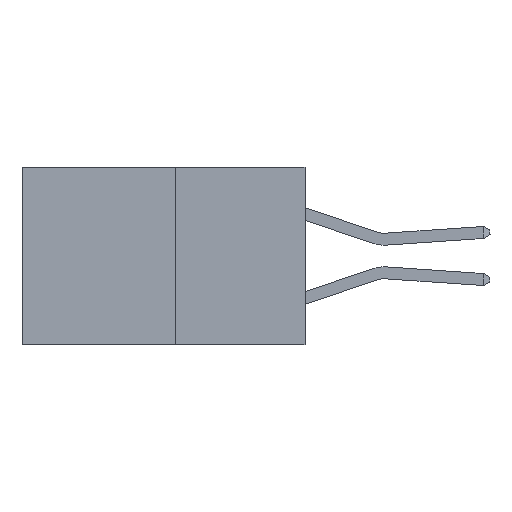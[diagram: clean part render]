
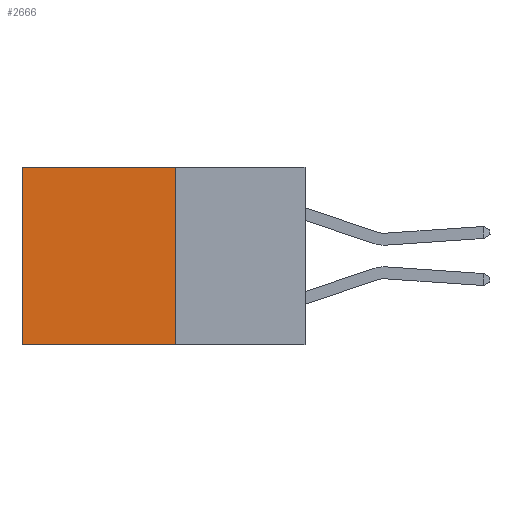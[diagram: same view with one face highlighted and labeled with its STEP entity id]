
A CAD part, left-side view. The second image highlights one B-rep face of the part: STEP entity #2666.
In plain terms, the highlighted planar face has unit normal (-1, 0, 0).
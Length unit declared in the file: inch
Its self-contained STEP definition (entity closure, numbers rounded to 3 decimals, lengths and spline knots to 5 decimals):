
#47 = CARTESIAN_POINT ( 'NONE',  ( 0.277, 0.27, -0.37 ) ) ;
#79 = CARTESIAN_POINT ( 'NONE',  ( 0.277, 0.27, -0.37 ) ) ;
#841 = LINE ( 'NONE', #14643, #8844 ) ;
#1040 = DIRECTION ( 'NONE',  ( 1., 0., 0. ) ) ;
#1284 = VERTEX_POINT ( 'NONE', #3802 ) ;
#1543 = VECTOR ( 'NONE', #5683, 39.37008 ) ;
#1975 = CARTESIAN_POINT ( 'NONE',  ( 0.277, 0.59, -0.37 ) ) ;
#2591 = ORIENTED_EDGE ( 'NONE', *, *, #8512, .T. ) ;
#2666 = ADVANCED_FACE ( 'NONE', ( #12675 ), #11684, .F. ) ;
#3070 = ORIENTED_EDGE ( 'NONE', *, *, #3448, .T. ) ;
#3448 = EDGE_CURVE ( 'NONE', #5344, #10267, #841, .T. ) ;
#3766 = AXIS2_PLACEMENT_3D ( 'NONE', #79, #1040, #9402 ) ;
#3802 = CARTESIAN_POINT ( 'NONE',  ( 0.277, 0.27, -0.37 ) ) ;
#4565 = LINE ( 'NONE', #11396, #1543 ) ;
#5344 = VERTEX_POINT ( 'NONE', #12441 ) ;
#5683 = DIRECTION ( 'NONE',  ( 0., 1., 0. ) ) ;
#6112 = LINE ( 'NONE', #9180, #11846 ) ;
#7127 = VECTOR ( 'NONE', #11447, 39.37008 ) ;
#8512 = EDGE_CURVE ( 'NONE', #14527, #5344, #4565, .T. ) ;
#8759 = EDGE_LOOP ( 'NONE', ( #3070, #11027, #10737, #2591 ) ) ;
#8844 = VECTOR ( 'NONE', #14381, 39.37008 ) ;
#9180 = CARTESIAN_POINT ( 'NONE',  ( 0.277, 0.27, -0.37 ) ) ;
#9402 = DIRECTION ( 'NONE',  ( 0., 0., -1. ) ) ;
#10267 = VERTEX_POINT ( 'NONE', #1975 ) ;
#10523 = EDGE_CURVE ( 'NONE', #1284, #10267, #6112, .T. ) ;
#10737 = ORIENTED_EDGE ( 'NONE', *, *, #13861, .F. ) ;
#11027 = ORIENTED_EDGE ( 'NONE', *, *, #10523, .F. ) ;
#11396 = CARTESIAN_POINT ( 'NONE',  ( 0.277, 0.27, 0. ) ) ;
#11447 = DIRECTION ( 'NONE',  ( 0., 0., -1. ) ) ;
#11496 = DIRECTION ( 'NONE',  ( 0., 1., 0. ) ) ;
#11684 = PLANE ( 'NONE',  #3766 ) ;
#11846 = VECTOR ( 'NONE', #11496, 39.37008 ) ;
#12441 = CARTESIAN_POINT ( 'NONE',  ( 0.277, 0.59, 0. ) ) ;
#12675 = FACE_OUTER_BOUND ( 'NONE', #8759, .T. ) ;
#12882 = LINE ( 'NONE', #47, #7127 ) ;
#13717 = CARTESIAN_POINT ( 'NONE',  ( 0.277, 0.27, 0. ) ) ;
#13861 = EDGE_CURVE ( 'NONE', #14527, #1284, #12882, .T. ) ;
#14381 = DIRECTION ( 'NONE',  ( 0., 0., -1. ) ) ;
#14527 = VERTEX_POINT ( 'NONE', #13717 ) ;
#14643 = CARTESIAN_POINT ( 'NONE',  ( 0.277, 0.59, -0.37 ) ) ;
